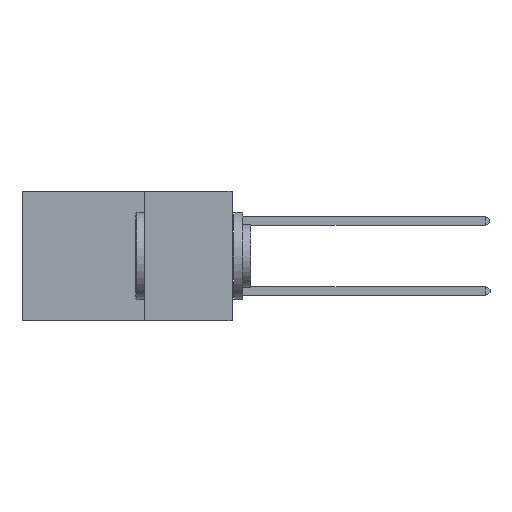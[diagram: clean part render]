
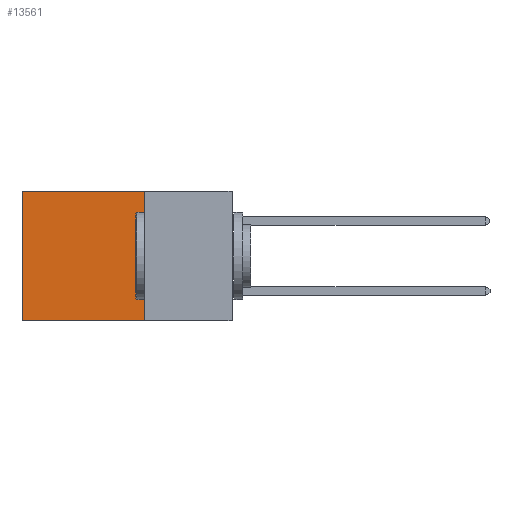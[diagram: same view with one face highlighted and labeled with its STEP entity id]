
A CAD part, left-side view. The second image highlights one B-rep face of the part: STEP entity #13561.
In plain terms, the highlighted planar face has unit normal (-1, 0, 0).
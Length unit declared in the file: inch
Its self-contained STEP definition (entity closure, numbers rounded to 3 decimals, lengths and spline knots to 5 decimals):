
#1038 = DIRECTION ( 'NONE',  ( 0., 0., -1. ) ) ;
#2664 = VERTEX_POINT ( 'NONE', #11121 ) ;
#2824 = LINE ( 'NONE', #21191, #7685 ) ;
#2852 = ORIENTED_EDGE ( 'NONE', *, *, #12678, .F. ) ;
#2952 = VERTEX_POINT ( 'NONE', #12892 ) ;
#4095 = AXIS2_PLACEMENT_3D ( 'NONE', #19253, #8910, #20971 ) ;
#4251 = VECTOR ( 'NONE', #1038, 39.37008 ) ;
#4928 = EDGE_CURVE ( 'NONE', #2664, #5361, #13687, .T. ) ;
#5279 = EDGE_LOOP ( 'NONE', ( #22247, #2852, #6255, #14950 ) ) ;
#5361 = VERTEX_POINT ( 'NONE', #7846 ) ;
#6255 = ORIENTED_EDGE ( 'NONE', *, *, #21830, .F. ) ;
#7451 = LINE ( 'NONE', #7596, #15680 ) ;
#7596 = CARTESIAN_POINT ( 'NONE',  ( 0.2875, 0.25, 0. ) ) ;
#7685 = VECTOR ( 'NONE', #10889, 39.37008 ) ;
#7846 = CARTESIAN_POINT ( 'NONE',  ( 0.2875, 0.6, -0.37 ) ) ;
#8627 = DIRECTION ( 'NONE',  ( 0., 0., -1. ) ) ;
#8910 = DIRECTION ( 'NONE',  ( 1., 0., 0. ) ) ;
#10238 = VECTOR ( 'NONE', #8627, 39.37008 ) ;
#10889 = DIRECTION ( 'NONE',  ( 0., 1., 0. ) ) ;
#11121 = CARTESIAN_POINT ( 'NONE',  ( 0.2875, 0.6, 0. ) ) ;
#11632 = EDGE_CURVE ( 'NONE', #15245, #2664, #7451, .T. ) ;
#11908 = CARTESIAN_POINT ( 'NONE',  ( 0.2875, 0.6, 0. ) ) ;
#12086 = CARTESIAN_POINT ( 'NONE',  ( 0.2875, 0.25, 0. ) ) ;
#12678 = EDGE_CURVE ( 'NONE', #2952, #5361, #2824, .T. ) ;
#12892 = CARTESIAN_POINT ( 'NONE',  ( 0.2875, 0.25, -0.37 ) ) ;
#13561 = ADVANCED_FACE ( 'NONE', ( #16901 ), #15836, .F. ) ;
#13687 = LINE ( 'NONE', #11908, #4251 ) ;
#14950 = ORIENTED_EDGE ( 'NONE', *, *, #11632, .T. ) ;
#15245 = VERTEX_POINT ( 'NONE', #12086 ) ;
#15680 = VECTOR ( 'NONE', #16384, 39.37008 ) ;
#15836 = PLANE ( 'NONE',  #4095 ) ;
#16384 = DIRECTION ( 'NONE',  ( 0., 1., 0. ) ) ;
#16901 = FACE_OUTER_BOUND ( 'NONE', #5279, .T. ) ;
#17275 = CARTESIAN_POINT ( 'NONE',  ( 0.2875, 0.25, 0. ) ) ;
#19253 = CARTESIAN_POINT ( 'NONE',  ( 0.2875, 0.25, 0. ) ) ;
#19396 = LINE ( 'NONE', #17275, #10238 ) ;
#20971 = DIRECTION ( 'NONE',  ( 0., 0., -1. ) ) ;
#21191 = CARTESIAN_POINT ( 'NONE',  ( 0.2875, 0.25, -0.37 ) ) ;
#21830 = EDGE_CURVE ( 'NONE', #15245, #2952, #19396, .T. ) ;
#22247 = ORIENTED_EDGE ( 'NONE', *, *, #4928, .T. ) ;
